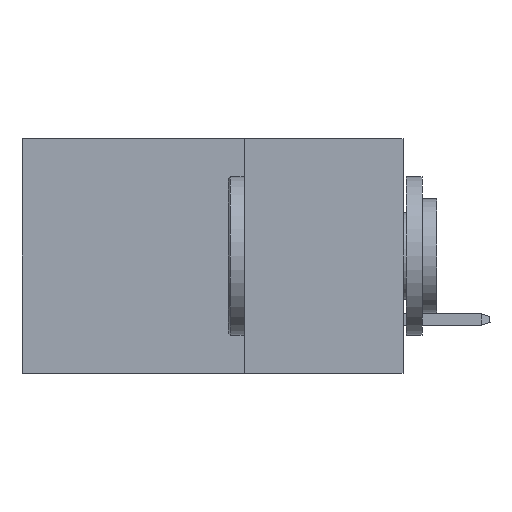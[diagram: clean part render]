
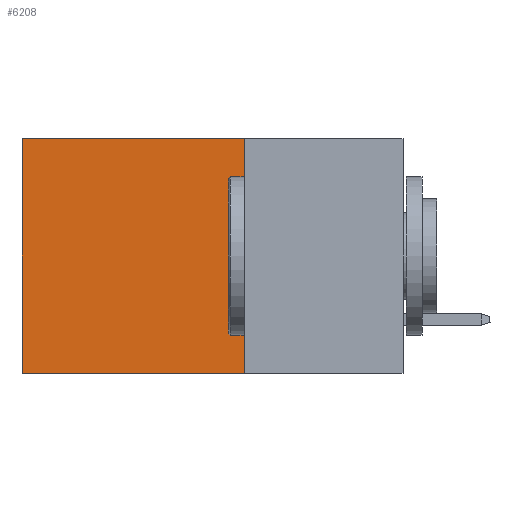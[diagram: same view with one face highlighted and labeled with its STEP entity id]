
A CAD part, left-side view. The second image highlights one B-rep face of the part: STEP entity #6208.
In plain terms, the highlighted planar face has unit normal (-1, 0, 0).
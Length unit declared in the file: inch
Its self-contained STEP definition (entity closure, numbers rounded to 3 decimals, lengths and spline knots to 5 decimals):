
#86 = AXIS2_PLACEMENT_3D ( 'NONE', #23372, #32005, #26079 ) ;
#542 = FACE_OUTER_BOUND ( 'NONE', #23589, .T. ) ;
#891 = DIRECTION ( 'NONE',  ( 0., 1., 0. ) ) ;
#1437 = EDGE_CURVE ( 'NONE', #7637, #10293, #21395, .T. ) ;
#3283 = CARTESIAN_POINT ( 'NONE',  ( 0.2875, 0.6, 0. ) ) ;
#4380 = CARTESIAN_POINT ( 'NONE',  ( 0.2875, 0.6, -0.37 ) ) ;
#6208 = ADVANCED_FACE ( 'NONE', ( #542 ), #11684, .F. ) ;
#6235 = DIRECTION ( 'NONE',  ( 0., 0., -1. ) ) ;
#6437 = DIRECTION ( 'NONE',  ( 0., 0., -1. ) ) ;
#7637 = VERTEX_POINT ( 'NONE', #3283 ) ;
#7780 = VERTEX_POINT ( 'NONE', #17027 ) ;
#9718 = CARTESIAN_POINT ( 'NONE',  ( 0.2875, 0.25, -0.37 ) ) ;
#10293 = VERTEX_POINT ( 'NONE', #4380 ) ;
#11684 = PLANE ( 'NONE',  #86 ) ;
#12006 = LINE ( 'NONE', #30197, #19829 ) ;
#12049 = CARTESIAN_POINT ( 'NONE',  ( 0.2875, 0.25, 0. ) ) ;
#16001 = VERTEX_POINT ( 'NONE', #36882 ) ;
#17027 = CARTESIAN_POINT ( 'NONE',  ( 0.2875, 0.25, 0. ) ) ;
#17437 = VECTOR ( 'NONE', #6437, 39.37008 ) ;
#19829 = VECTOR ( 'NONE', #6235, 39.37008 ) ;
#21395 = LINE ( 'NONE', #35761, #17437 ) ;
#23372 = CARTESIAN_POINT ( 'NONE',  ( 0.2875, 0.25, 0. ) ) ;
#23589 = EDGE_LOOP ( 'NONE', ( #29138, #37727, #31962, #36839 ) ) ;
#24121 = VECTOR ( 'NONE', #891, 39.37008 ) ;
#26079 = DIRECTION ( 'NONE',  ( 0., 0., -1. ) ) ;
#26638 = EDGE_CURVE ( 'NONE', #16001, #10293, #33490, .T. ) ;
#29138 = ORIENTED_EDGE ( 'NONE', *, *, #1437, .T. ) ;
#29483 = LINE ( 'NONE', #12049, #32253 ) ;
#30197 = CARTESIAN_POINT ( 'NONE',  ( 0.2875, 0.25, 0. ) ) ;
#31382 = EDGE_CURVE ( 'NONE', #7780, #16001, #12006, .T. ) ;
#31962 = ORIENTED_EDGE ( 'NONE', *, *, #31382, .F. ) ;
#32005 = DIRECTION ( 'NONE',  ( 1., 0., 0. ) ) ;
#32253 = VECTOR ( 'NONE', #35422, 39.37008 ) ;
#33490 = LINE ( 'NONE', #9718, #24121 ) ;
#35422 = DIRECTION ( 'NONE',  ( 0., 1., 0. ) ) ;
#35750 = EDGE_CURVE ( 'NONE', #7780, #7637, #29483, .T. ) ;
#35761 = CARTESIAN_POINT ( 'NONE',  ( 0.2875, 0.6, 0. ) ) ;
#36839 = ORIENTED_EDGE ( 'NONE', *, *, #35750, .T. ) ;
#36882 = CARTESIAN_POINT ( 'NONE',  ( 0.2875, 0.25, -0.37 ) ) ;
#37727 = ORIENTED_EDGE ( 'NONE', *, *, #26638, .F. ) ;
